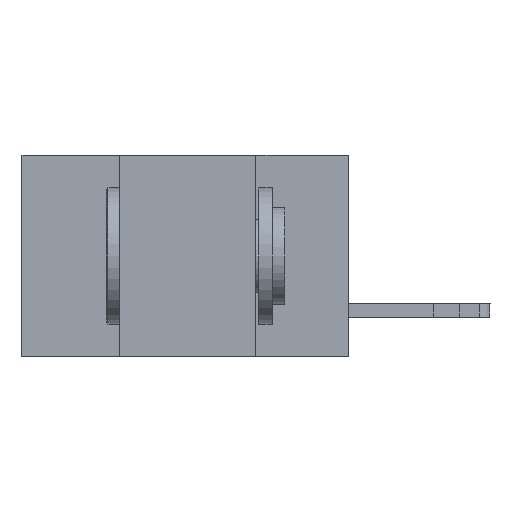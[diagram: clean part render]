
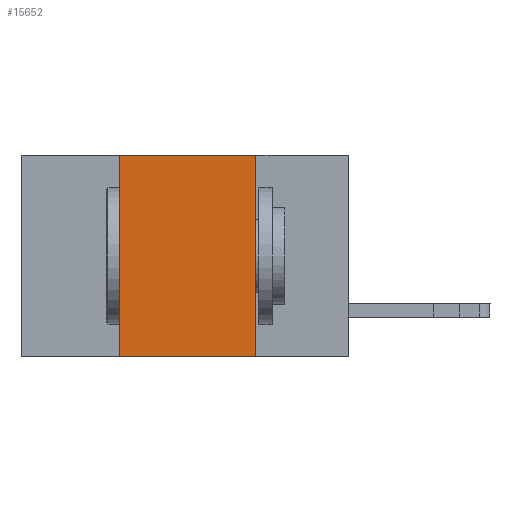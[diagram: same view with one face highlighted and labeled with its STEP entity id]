
A CAD part, left-side view. The second image highlights one B-rep face of the part: STEP entity #15652.
In plain terms, the highlighted planar face has unit normal (-1, 0, 0).
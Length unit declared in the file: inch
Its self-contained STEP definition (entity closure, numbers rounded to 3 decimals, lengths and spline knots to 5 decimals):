
#140 = EDGE_CURVE ( 'NONE', #3951, #3042, #14145, .T. ) ;
#348 = VECTOR ( 'NONE', #16553, 39.37008 ) ;
#432 = CARTESIAN_POINT ( 'NONE',  ( 0., 0.6, 0. ) ) ;
#460 = VERTEX_POINT ( 'NONE', #11584 ) ;
#618 = VECTOR ( 'NONE', #5710, 39.37008 ) ;
#648 = VERTEX_POINT ( 'NONE', #2361 ) ;
#775 = ORIENTED_EDGE ( 'NONE', *, *, #140, .F. ) ;
#828 = PLANE ( 'NONE',  #12406 ) ;
#904 = DIRECTION ( 'NONE',  ( 0., 0., -1. ) ) ;
#2358 = DIRECTION ( 'NONE',  ( 1., 0., 0. ) ) ;
#2361 = CARTESIAN_POINT ( 'NONE',  ( 0., 0.42, -0.37 ) ) ;
#2490 = CARTESIAN_POINT ( 'NONE',  ( 0., 0.42, 0. ) ) ;
#2991 = ORIENTED_EDGE ( 'NONE', *, *, #16605, .F. ) ;
#3042 = VERTEX_POINT ( 'NONE', #11778 ) ;
#3951 = VERTEX_POINT ( 'NONE', #6430 ) ;
#5710 = DIRECTION ( 'NONE',  ( 0., 0., -1. ) ) ;
#5925 = DIRECTION ( 'NONE',  ( 0., -1., 0. ) ) ;
#6257 = ORIENTED_EDGE ( 'NONE', *, *, #17620, .F. ) ;
#6430 = CARTESIAN_POINT ( 'NONE',  ( 0., 0.42, 0. ) ) ;
#7494 = CARTESIAN_POINT ( 'NONE',  ( 0., 0.17, 0. ) ) ;
#7865 = EDGE_CURVE ( 'NONE', #648, #460, #11311, .T. ) ;
#8956 = DIRECTION ( 'NONE',  ( 0., -1., 0. ) ) ;
#11311 = LINE ( 'NONE', #14298, #12278 ) ;
#11584 = CARTESIAN_POINT ( 'NONE',  ( 0., 0.17, -0.37 ) ) ;
#11778 = CARTESIAN_POINT ( 'NONE',  ( 0., 0.17, 0. ) ) ;
#12255 = ORIENTED_EDGE ( 'NONE', *, *, #7865, .T. ) ;
#12278 = VECTOR ( 'NONE', #8956, 39.37008 ) ;
#12355 = EDGE_LOOP ( 'NONE', ( #2991, #775, #6257, #12255 ) ) ;
#12406 = AXIS2_PLACEMENT_3D ( 'NONE', #14636, #2358, #904 ) ;
#13098 = VECTOR ( 'NONE', #5925, 39.37008 ) ;
#13189 = FACE_OUTER_BOUND ( 'NONE', #12355, .T. ) ;
#14145 = LINE ( 'NONE', #432, #13098 ) ;
#14298 = CARTESIAN_POINT ( 'NONE',  ( 0., 0.6, -0.37 ) ) ;
#14636 = CARTESIAN_POINT ( 'NONE',  ( 0., 0.6, 0. ) ) ;
#14839 = LINE ( 'NONE', #2490, #348 ) ;
#15652 = ADVANCED_FACE ( 'NONE', ( #13189 ), #828, .F. ) ;
#16553 = DIRECTION ( 'NONE',  ( 0., 0., 1. ) ) ;
#16605 = EDGE_CURVE ( 'NONE', #3042, #460, #16981, .T. ) ;
#16981 = LINE ( 'NONE', #7494, #618 ) ;
#17620 = EDGE_CURVE ( 'NONE', #648, #3951, #14839, .T. ) ;
